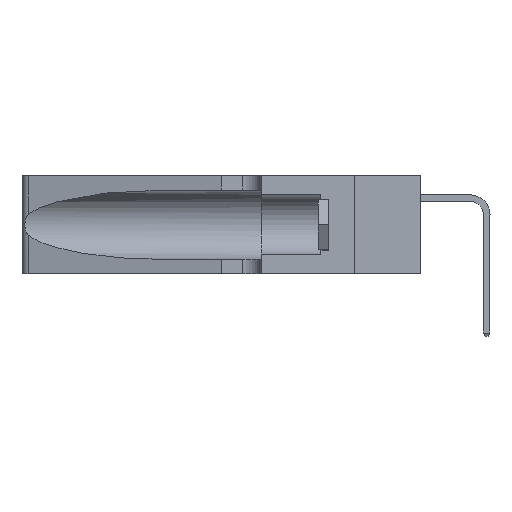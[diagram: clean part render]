
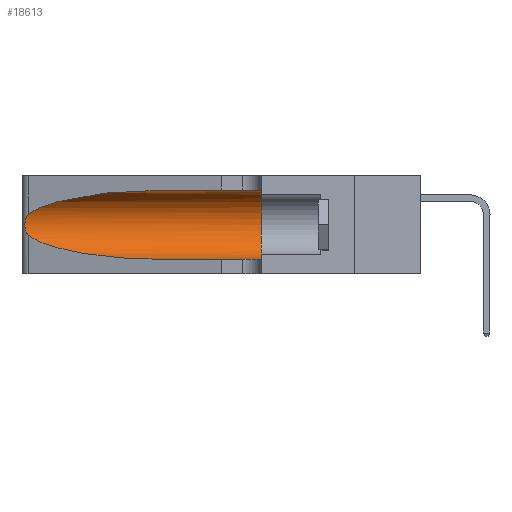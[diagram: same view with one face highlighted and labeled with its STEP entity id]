
A CAD part, left-side view. The second image highlights one B-rep face of the part: STEP entity #18613.
In plain terms, the highlighted cylindrical face has radius 3.308 mm (diameter 6.617 mm), a partial arc.
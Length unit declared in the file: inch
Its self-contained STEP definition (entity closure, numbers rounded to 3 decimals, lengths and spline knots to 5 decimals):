
#728 = CARTESIAN_POINT ( 'NONE',  ( 0.1305, 1.61858, 0.31525 ) ) ;
#1276 =( BOUNDED_CURVE ( )  B_SPLINE_CURVE ( 3, ( #30495, #20933, #11303, #28181 ),
 .UNSPECIFIED., .F., .F. ) 
 B_SPLINE_CURVE_WITH_KNOTS ( ( 4, 4 ),
 ( 3.44316, 4.71239 ),
 .UNSPECIFIED. ) 
 CURVE ( )  GEOMETRIC_REPRESENTATION_ITEM ( )  RATIONAL_B_SPLINE_CURVE ( ( 1., 0.87, 0.87, 1. ) ) 
 REPRESENTATION_ITEM ( '' )  );
#1298 = DIRECTION ( 'NONE',  ( 0., 1., 0. ) ) ;
#2042 = VERTEX_POINT ( 'NONE', #3324 ) ;
#2352 = CARTESIAN_POINT ( 'NONE',  ( 0.26017, 1.23833, 0.17102 ) ) ;
#2427 = CARTESIAN_POINT ( 'NONE',  ( 0.2373, 1.15595, 0.28018 ) ) ;
#3147 = EDGE_LOOP ( 'NONE', ( #27846, #3243, #14505, #4894, #5258, #30899 ) ) ;
#3243 = ORIENTED_EDGE ( 'NONE', *, *, #15931, .T. ) ;
#3324 = CARTESIAN_POINT ( 'NONE',  ( 0.25487, 1.22718, 0.22369 ) ) ;
#4779 = CARTESIAN_POINT ( 'NONE',  ( 0.25789, 1.23486, 0.15765 ) ) ;
#4894 = ORIENTED_EDGE ( 'NONE', *, *, #22973, .T. ) ;
#5258 = ORIENTED_EDGE ( 'NONE', *, *, #30878, .F. ) ;
#6539 = EDGE_CURVE ( 'NONE', #27571, #27577, #17907, .T. ) ;
#6728 = CIRCLE ( 'NONE', #25317, 0.13025 ) ;
#6898 = B_SPLINE_CURVE_WITH_KNOTS ( 'NONE', 3,
 ( #21660, #16813, #26506, #12048, #28896, #14500, #31334, #16922, #2352, #19351, #4779, #21763, #7216, #24193 ),
 .UNSPECIFIED., .F., .F.,
 ( 4, 2, 2, 2, 2, 2, 4 ),
 ( 0., 0.00027, 0.00053, 0.00107, 0.0016, 0.00187, 0.00214 ),
 .UNSPECIFIED. ) ;
#7216 = CARTESIAN_POINT ( 'NONE',  ( 0.25555, 1.22993, 0.14849 ) ) ;
#8360 = CYLINDRICAL_SURFACE ( 'NONE', #9573, 0.13025 ) ;
#9573 = AXIS2_PLACEMENT_3D ( 'NONE', #29999, #15601, #10705 ) ;
#9663 = CARTESIAN_POINT ( 'NONE',  ( 0.18966, 0.96281, 0.31525 ) ) ;
#9874 = EDGE_CURVE ( 'NONE', #27571, #2042, #15006, .T. ) ;
#10705 = DIRECTION ( 'NONE',  ( 0., 0., -1. ) ) ;
#11303 = CARTESIAN_POINT ( 'NONE',  ( 0.18966, 0.96281, 0.05475 ) ) ;
#12048 = CARTESIAN_POINT ( 'NONE',  ( 0.25787, 1.23484, 0.2124 ) ) ;
#12124 = CARTESIAN_POINT ( 'NONE',  ( 0.1305, 0.72297, 0.31525 ) ) ;
#12512 = CARTESIAN_POINT ( 'NONE',  ( 0.1305, 0.35, 0.31525 ) ) ;
#12888 = DIRECTION ( 'NONE',  ( 0., -1., 0. ) ) ;
#13555 = CARTESIAN_POINT ( 'NONE',  ( 0.25487, 1.22718, 0.14631 ) ) ;
#14500 = CARTESIAN_POINT ( 'NONE',  ( 0.26018, 1.23835, 0.19895 ) ) ;
#14505 = ORIENTED_EDGE ( 'NONE', *, *, #25256, .T. ) ;
#14959 = CARTESIAN_POINT ( 'NONE',  ( 0.1305, 0.72297, 0.31525 ) ) ;
#15006 =( BOUNDED_CURVE ( )  B_SPLINE_CURVE ( 3, ( #12124, #9663, #2427, #19429 ),
 .UNSPECIFIED., .F., .F. ) 
 B_SPLINE_CURVE_WITH_KNOTS ( ( 4, 4 ),
 ( 1.5708, 2.84003 ),
 .UNSPECIFIED. ) 
 CURVE ( )  GEOMETRIC_REPRESENTATION_ITEM ( )  RATIONAL_B_SPLINE_CURVE ( ( 1., 0.87, 0.87, 1. ) ) 
 REPRESENTATION_ITEM ( '' )  );
#15601 = DIRECTION ( 'NONE',  ( 0., -1., 0. ) ) ;
#15880 = CARTESIAN_POINT ( 'NONE',  ( 0.1305, 0.35, 0.185 ) ) ;
#15931 = EDGE_CURVE ( 'NONE', #2042, #18721, #6898, .T. ) ;
#16813 = CARTESIAN_POINT ( 'NONE',  ( 0.25555, 1.22994, 0.2215 ) ) ;
#16922 = CARTESIAN_POINT ( 'NONE',  ( 0.26075, 1.23896, 0.178 ) ) ;
#16974 = VERTEX_POINT ( 'NONE', #25607 ) ;
#17847 = CARTESIAN_POINT ( 'NONE',  ( 0.1305, 0.72297, 0.05475 ) ) ;
#17907 = LINE ( 'NONE', #728, #18669 ) ;
#18315 = DIRECTION ( 'NONE',  ( 0., 0., 1. ) ) ;
#18613 = ADVANCED_FACE ( 'NONE', ( #27686 ), #8360, .F. ) ;
#18669 = VECTOR ( 'NONE', #12888, 39.37008 ) ;
#18721 = VERTEX_POINT ( 'NONE', #13555 ) ;
#19351 = CARTESIAN_POINT ( 'NONE',  ( 0.25856, 1.23593, 0.16098 ) ) ;
#19429 = CARTESIAN_POINT ( 'NONE',  ( 0.25487, 1.22718, 0.22369 ) ) ;
#19886 = VERTEX_POINT ( 'NONE', #17847 ) ;
#20933 = CARTESIAN_POINT ( 'NONE',  ( 0.2373, 1.15595, 0.08982 ) ) ;
#21660 = CARTESIAN_POINT ( 'NONE',  ( 0.25487, 1.22718, 0.22369 ) ) ;
#21763 = CARTESIAN_POINT ( 'NONE',  ( 0.25639, 1.23186, 0.15144 ) ) ;
#22036 = CARTESIAN_POINT ( 'NONE',  ( 0.1305, 1.61858, 0.05475 ) ) ;
#22973 = EDGE_CURVE ( 'NONE', #19886, #16974, #27336, .T. ) ;
#24193 = CARTESIAN_POINT ( 'NONE',  ( 0.25487, 1.22718, 0.14631 ) ) ;
#24445 = DIRECTION ( 'NONE',  ( 0., -1., 0. ) ) ;
#25256 = EDGE_CURVE ( 'NONE', #18721, #19886, #1276, .T. ) ;
#25317 = AXIS2_PLACEMENT_3D ( 'NONE', #15880, #1298, #18315 ) ;
#25607 = CARTESIAN_POINT ( 'NONE',  ( 0.1305, 0.35, 0.05475 ) ) ;
#26506 = CARTESIAN_POINT ( 'NONE',  ( 0.25639, 1.23184, 0.21858 ) ) ;
#27336 = LINE ( 'NONE', #22036, #28094 ) ;
#27571 = VERTEX_POINT ( 'NONE', #14959 ) ;
#27577 = VERTEX_POINT ( 'NONE', #12512 ) ;
#27686 = FACE_OUTER_BOUND ( 'NONE', #3147, .T. ) ;
#27846 = ORIENTED_EDGE ( 'NONE', *, *, #9874, .T. ) ;
#28094 = VECTOR ( 'NONE', #24445, 39.37008 ) ;
#28181 = CARTESIAN_POINT ( 'NONE',  ( 0.1305, 0.72297, 0.05475 ) ) ;
#28896 = CARTESIAN_POINT ( 'NONE',  ( 0.25854, 1.2359, 0.20912 ) ) ;
#29999 = CARTESIAN_POINT ( 'NONE',  ( 0.1305, 1.61858, 0.185 ) ) ;
#30495 = CARTESIAN_POINT ( 'NONE',  ( 0.25487, 1.22718, 0.14631 ) ) ;
#30878 = EDGE_CURVE ( 'NONE', #27577, #16974, #6728, .T. ) ;
#30899 = ORIENTED_EDGE ( 'NONE', *, *, #6539, .F. ) ;
#31334 = CARTESIAN_POINT ( 'NONE',  ( 0.26075, 1.23896, 0.19203 ) ) ;
